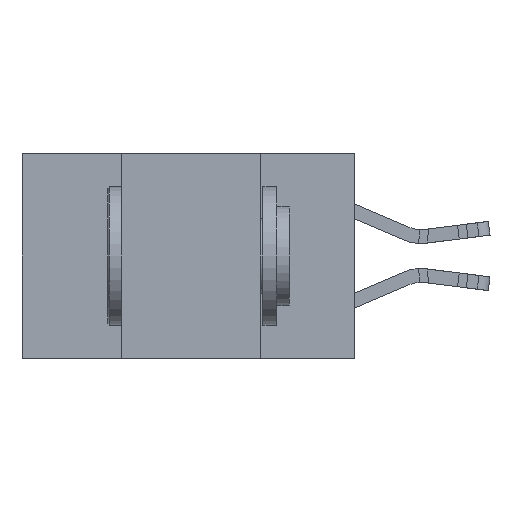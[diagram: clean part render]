
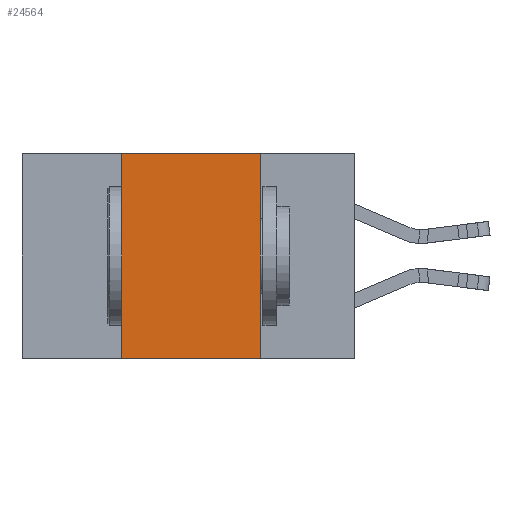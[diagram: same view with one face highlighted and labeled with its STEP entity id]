
A CAD part, left-side view. The second image highlights one B-rep face of the part: STEP entity #24564.
In plain terms, the highlighted planar face has unit normal (-1, 0, 0).
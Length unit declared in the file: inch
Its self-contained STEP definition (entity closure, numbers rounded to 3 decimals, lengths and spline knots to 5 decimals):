
#1240 = EDGE_CURVE ( 'NONE', #30728, #24748, #23323, .T. ) ;
#1273 = CARTESIAN_POINT ( 'NONE',  ( 0., 0.17, -0.37 ) ) ;
#2130 = CARTESIAN_POINT ( 'NONE',  ( 0., 0.42, 0. ) ) ;
#3240 = DIRECTION ( 'NONE',  ( 1., 0., 0. ) ) ;
#3533 = EDGE_CURVE ( 'NONE', #4417, #15241, #7858, .T. ) ;
#3750 = ORIENTED_EDGE ( 'NONE', *, *, #12760, .F. ) ;
#4417 = VERTEX_POINT ( 'NONE', #9925 ) ;
#4580 = VECTOR ( 'NONE', #22217, 39.37008 ) ;
#4979 = CARTESIAN_POINT ( 'NONE',  ( 0., 0.6, -0.37 ) ) ;
#7858 = LINE ( 'NONE', #16186, #20095 ) ;
#8685 = DIRECTION ( 'NONE',  ( 0., 0., 1. ) ) ;
#9925 = CARTESIAN_POINT ( 'NONE',  ( 0., 0.42, -0.37 ) ) ;
#12760 = EDGE_CURVE ( 'NONE', #15241, #30728, #14781, .T. ) ;
#13350 = CARTESIAN_POINT ( 'NONE',  ( 0., 0.17, 0. ) ) ;
#13608 = CARTESIAN_POINT ( 'NONE',  ( 0., 0.6, 0. ) ) ;
#14781 = LINE ( 'NONE', #13608, #25406 ) ;
#15241 = VERTEX_POINT ( 'NONE', #2130 ) ;
#15323 = VECTOR ( 'NONE', #29575, 39.37008 ) ;
#16186 = CARTESIAN_POINT ( 'NONE',  ( 0., 0.42, 0. ) ) ;
#16939 = EDGE_LOOP ( 'NONE', ( #21044, #3750, #21439, #18007 ) ) ;
#17664 = LINE ( 'NONE', #4979, #4580 ) ;
#17979 = CARTESIAN_POINT ( 'NONE',  ( 0., 0.6, 0. ) ) ;
#18007 = ORIENTED_EDGE ( 'NONE', *, *, #24377, .T. ) ;
#18028 = FACE_OUTER_BOUND ( 'NONE', #16939, .T. ) ;
#20095 = VECTOR ( 'NONE', #8685, 39.37008 ) ;
#20167 = CARTESIAN_POINT ( 'NONE',  ( 0., 0.17, 0. ) ) ;
#20413 = DIRECTION ( 'NONE',  ( 0., 0., -1. ) ) ;
#21044 = ORIENTED_EDGE ( 'NONE', *, *, #1240, .F. ) ;
#21439 = ORIENTED_EDGE ( 'NONE', *, *, #3533, .F. ) ;
#22217 = DIRECTION ( 'NONE',  ( 0., -1., 0. ) ) ;
#23323 = LINE ( 'NONE', #20167, #15323 ) ;
#24377 = EDGE_CURVE ( 'NONE', #4417, #24748, #17664, .T. ) ;
#24564 = ADVANCED_FACE ( 'NONE', ( #18028 ), #27685, .F. ) ;
#24748 = VERTEX_POINT ( 'NONE', #1273 ) ;
#25406 = VECTOR ( 'NONE', #28166, 39.37008 ) ;
#27685 = PLANE ( 'NONE',  #29410 ) ;
#28166 = DIRECTION ( 'NONE',  ( 0., -1., 0. ) ) ;
#29410 = AXIS2_PLACEMENT_3D ( 'NONE', #17979, #3240, #20413 ) ;
#29575 = DIRECTION ( 'NONE',  ( 0., 0., -1. ) ) ;
#30728 = VERTEX_POINT ( 'NONE', #13350 ) ;
